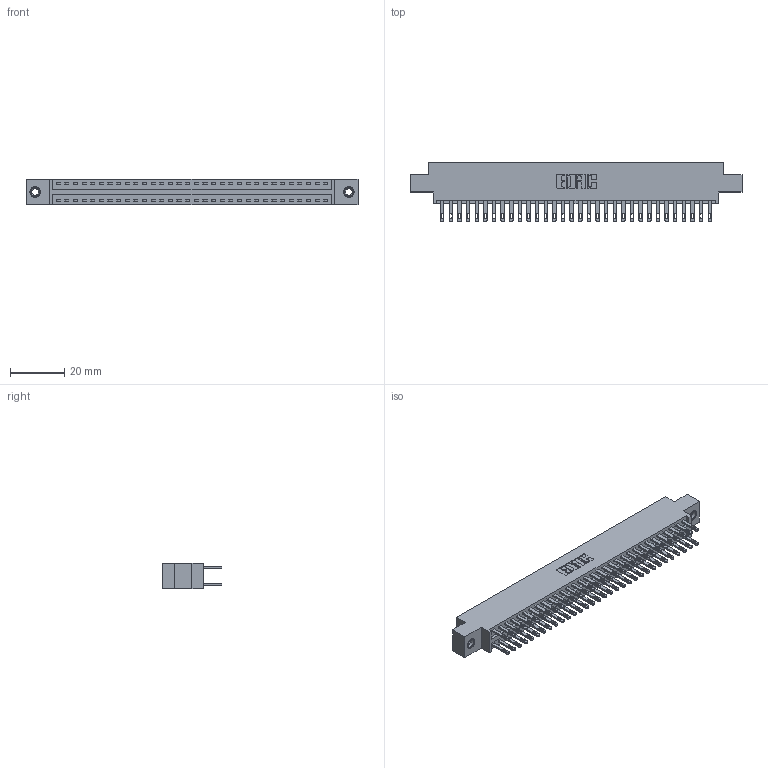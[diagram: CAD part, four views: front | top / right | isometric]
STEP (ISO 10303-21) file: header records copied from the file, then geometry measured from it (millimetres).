
FILE_DESCRIPTION (( 'STEP AP203' ), '1' );
FILE_NAME ('346-064-500-807.STEP', '2022-05-24T14:47:03', ( '' ), ( '' ), 'SwSTEP 2.0', 'SolidWorks 2020', '' );
FILE_SCHEMA (( 'CONFIG_CONTROL_DESIGN' ));
Length unit declared in the file: inch
Products named in the file (4): 345-292-001_345-293-100; 346-064-500-807; 345-250-001_345-250-005-103; 346 Part_0.170 Offset - 0.156 Dia-TI
Assembly tree (67 placements, depth 2):
  346-064-500-807
    346 Part_0.170 Offset - 0.156 Dia-TI
    345-292-001_345-293-100  x64
    345-250-001_345-250-005-103  x2
Bounding box: 122.17 x 21.84 x 9.4 mm (x, y, z)
Volume: 11863.3 mm3; surface area: 17032.9 mm2
Topology: 67 solids, 67 shells, 3258 faces, 9885 edges, 6582 vertices
Faces by surface type: plane 1968, cylinder 1274, cone 12, torus 4
Entity records: 23478 total; most frequent: CARTESIAN_POINT 3867, ORIENTED_EDGE 3794, DIRECTION 3487, EDGE_CURVE 1897, VECTOR 1613, LINE 1613, VERTEX_POINT 1260, AXIS2_PLACEMENT_3D 937
